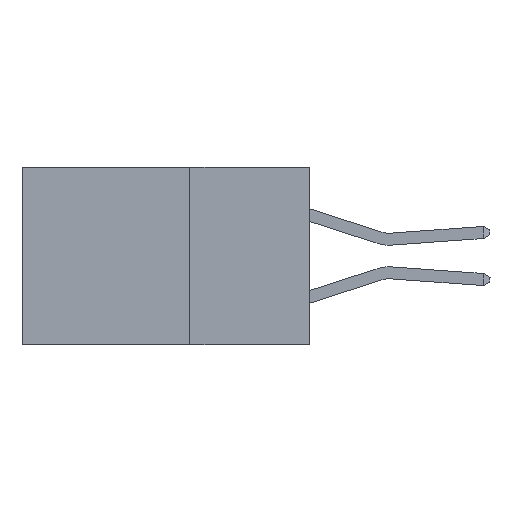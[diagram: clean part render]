
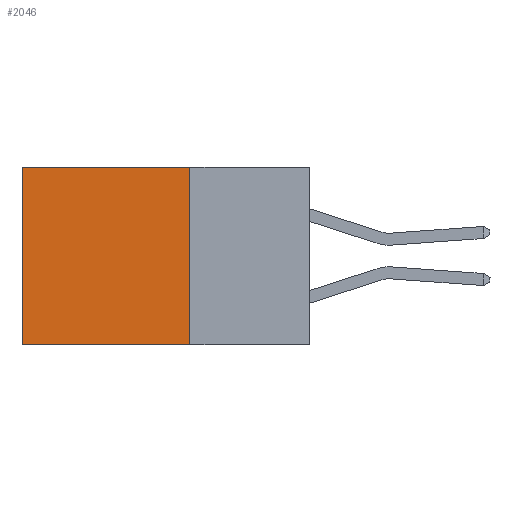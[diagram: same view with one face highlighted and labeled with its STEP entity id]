
A CAD part, left-side view. The second image highlights one B-rep face of the part: STEP entity #2046.
In plain terms, the highlighted planar face has unit normal (-1, 0, 0).
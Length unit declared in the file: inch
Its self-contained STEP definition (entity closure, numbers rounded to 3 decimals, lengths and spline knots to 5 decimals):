
#1135 = DIRECTION ( 'NONE',  ( 1., 0., 0. ) ) ;
#1179 = VERTEX_POINT ( 'NONE', #4458 ) ;
#1614 = DIRECTION ( 'NONE',  ( 0., 0., -1. ) ) ;
#2046 = ADVANCED_FACE ( 'NONE', ( #6025 ), #7773, .F. ) ;
#2260 = VECTOR ( 'NONE', #1614, 39.37008 ) ;
#4458 = CARTESIAN_POINT ( 'NONE',  ( 0.298, 0.6, -0.37 ) ) ;
#4663 = DIRECTION ( 'NONE',  ( 0., 0., -1. ) ) ;
#4672 = CARTESIAN_POINT ( 'NONE',  ( 0.298, 0.6, 0. ) ) ;
#4812 = LINE ( 'NONE', #9106, #10583 ) ;
#4876 = LINE ( 'NONE', #4987, #2260 ) ;
#4987 = CARTESIAN_POINT ( 'NONE',  ( 0.298, 0.6, 0. ) ) ;
#5304 = VECTOR ( 'NONE', #12408, 39.37008 ) ;
#5516 = CARTESIAN_POINT ( 'NONE',  ( 0.298, 0.25, 0. ) ) ;
#6025 = FACE_OUTER_BOUND ( 'NONE', #8619, .T. ) ;
#6030 = DIRECTION ( 'NONE',  ( 0., 1., 0. ) ) ;
#6209 = EDGE_CURVE ( 'NONE', #13955, #12608, #13902, .T. ) ;
#6512 = ORIENTED_EDGE ( 'NONE', *, *, #10840, .T. ) ;
#7021 = VERTEX_POINT ( 'NONE', #4672 ) ;
#7247 = AXIS2_PLACEMENT_3D ( 'NONE', #10088, #1135, #9982 ) ;
#7570 = LINE ( 'NONE', #10168, #5304 ) ;
#7773 = PLANE ( 'NONE',  #7247 ) ;
#8619 = EDGE_LOOP ( 'NONE', ( #9042, #13866, #10592, #6512 ) ) ;
#9042 = ORIENTED_EDGE ( 'NONE', *, *, #12966, .T. ) ;
#9106 = CARTESIAN_POINT ( 'NONE',  ( 0.298, 0.25, -0.37 ) ) ;
#9266 = CARTESIAN_POINT ( 'NONE',  ( 0.298, 0.25, 0. ) ) ;
#9982 = DIRECTION ( 'NONE',  ( 0., 0., -1. ) ) ;
#10088 = CARTESIAN_POINT ( 'NONE',  ( 0.298, 0.25, 0. ) ) ;
#10168 = CARTESIAN_POINT ( 'NONE',  ( 0.298, 0.25, 0. ) ) ;
#10232 = EDGE_CURVE ( 'NONE', #12608, #1179, #4812, .T. ) ;
#10583 = VECTOR ( 'NONE', #6030, 39.37008 ) ;
#10592 = ORIENTED_EDGE ( 'NONE', *, *, #6209, .F. ) ;
#10777 = CARTESIAN_POINT ( 'NONE',  ( 0.298, 0.25, -0.37 ) ) ;
#10840 = EDGE_CURVE ( 'NONE', #13955, #7021, #7570, .T. ) ;
#10951 = VECTOR ( 'NONE', #4663, 39.37008 ) ;
#12408 = DIRECTION ( 'NONE',  ( 0., 1., 0. ) ) ;
#12608 = VERTEX_POINT ( 'NONE', #10777 ) ;
#12966 = EDGE_CURVE ( 'NONE', #7021, #1179, #4876, .T. ) ;
#13866 = ORIENTED_EDGE ( 'NONE', *, *, #10232, .F. ) ;
#13902 = LINE ( 'NONE', #9266, #10951 ) ;
#13955 = VERTEX_POINT ( 'NONE', #5516 ) ;
